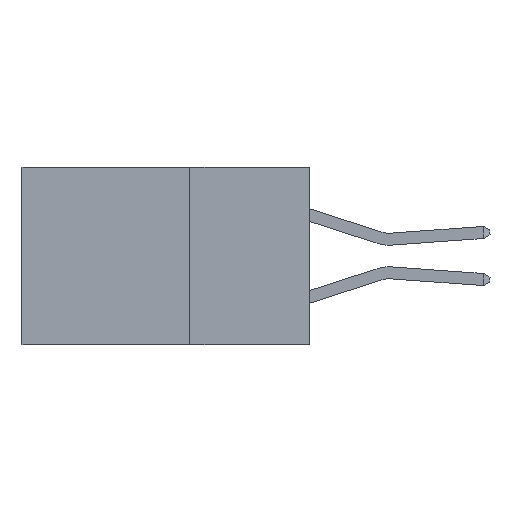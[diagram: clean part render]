
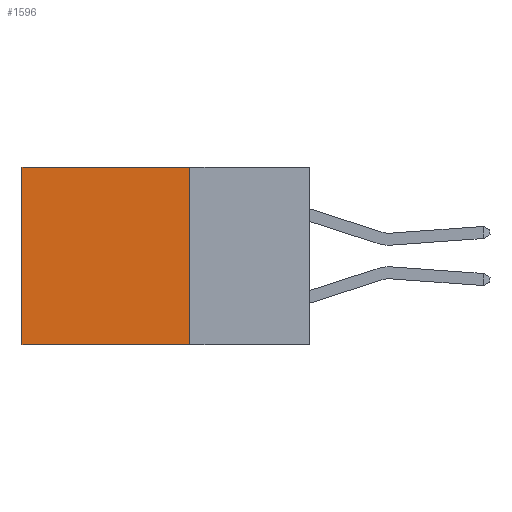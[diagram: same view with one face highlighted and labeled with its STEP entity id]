
A CAD part, left-side view. The second image highlights one B-rep face of the part: STEP entity #1596.
In plain terms, the highlighted planar face has unit normal (-1, 0, 0).
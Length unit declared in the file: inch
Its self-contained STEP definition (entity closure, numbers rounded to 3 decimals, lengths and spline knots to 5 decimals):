
#513 = VECTOR ( 'NONE', #1349, 39.37008 ) ;
#536 = DIRECTION ( 'NONE',  ( 0., 0., -1. ) ) ;
#1013 = VECTOR ( 'NONE', #536, 39.37008 ) ;
#1141 = CARTESIAN_POINT ( 'NONE',  ( 0.298, 0.6, 0. ) ) ;
#1349 = DIRECTION ( 'NONE',  ( 0., 1., 0. ) ) ;
#1370 = VERTEX_POINT ( 'NONE', #6317 ) ;
#1448 = ORIENTED_EDGE ( 'NONE', *, *, #3721, .T. ) ;
#1596 = ADVANCED_FACE ( 'NONE', ( #5621 ), #1990, .F. ) ;
#1723 = LINE ( 'NONE', #3719, #8048 ) ;
#1967 = CARTESIAN_POINT ( 'NONE',  ( 0.298, 0.6, -0.37 ) ) ;
#1990 = PLANE ( 'NONE',  #4408 ) ;
#2029 = DIRECTION ( 'NONE',  ( 0., 0., -1. ) ) ;
#2084 = DIRECTION ( 'NONE',  ( 1., 0., 0. ) ) ;
#2103 = CARTESIAN_POINT ( 'NONE',  ( 0.298, 0.25, -0.37 ) ) ;
#2775 = CARTESIAN_POINT ( 'NONE',  ( 0.298, 0.25, 0. ) ) ;
#3104 = DIRECTION ( 'NONE',  ( 0., 0., -1. ) ) ;
#3303 = LINE ( 'NONE', #1141, #1013 ) ;
#3368 = VERTEX_POINT ( 'NONE', #10455 ) ;
#3719 = CARTESIAN_POINT ( 'NONE',  ( 0.298, 0.25, 0. ) ) ;
#3721 = EDGE_CURVE ( 'NONE', #1370, #9197, #6247, .T. ) ;
#4277 = EDGE_CURVE ( 'NONE', #3368, #5827, #6877, .T. ) ;
#4408 = AXIS2_PLACEMENT_3D ( 'NONE', #7682, #2084, #3104 ) ;
#4788 = EDGE_CURVE ( 'NONE', #1370, #3368, #1723, .T. ) ;
#5621 = FACE_OUTER_BOUND ( 'NONE', #6065, .T. ) ;
#5827 = VERTEX_POINT ( 'NONE', #1967 ) ;
#5926 = EDGE_CURVE ( 'NONE', #9197, #5827, #3303, .T. ) ;
#5933 = ORIENTED_EDGE ( 'NONE', *, *, #5926, .T. ) ;
#6065 = EDGE_LOOP ( 'NONE', ( #5933, #8672, #7256, #1448 ) ) ;
#6247 = LINE ( 'NONE', #2775, #7943 ) ;
#6317 = CARTESIAN_POINT ( 'NONE',  ( 0.298, 0.25, 0. ) ) ;
#6877 = LINE ( 'NONE', #2103, #513 ) ;
#7256 = ORIENTED_EDGE ( 'NONE', *, *, #4788, .F. ) ;
#7337 = DIRECTION ( 'NONE',  ( 0., 1., 0. ) ) ;
#7682 = CARTESIAN_POINT ( 'NONE',  ( 0.298, 0.25, 0. ) ) ;
#7943 = VECTOR ( 'NONE', #7337, 39.37008 ) ;
#8048 = VECTOR ( 'NONE', #2029, 39.37008 ) ;
#8672 = ORIENTED_EDGE ( 'NONE', *, *, #4277, .F. ) ;
#9125 = CARTESIAN_POINT ( 'NONE',  ( 0.298, 0.6, 0. ) ) ;
#9197 = VERTEX_POINT ( 'NONE', #9125 ) ;
#10455 = CARTESIAN_POINT ( 'NONE',  ( 0.298, 0.25, -0.37 ) ) ;
